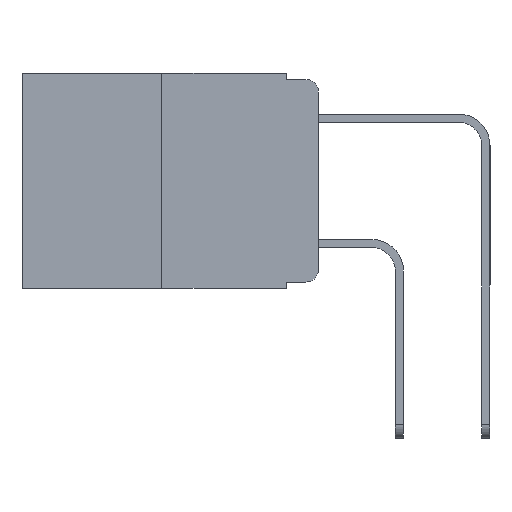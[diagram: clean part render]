
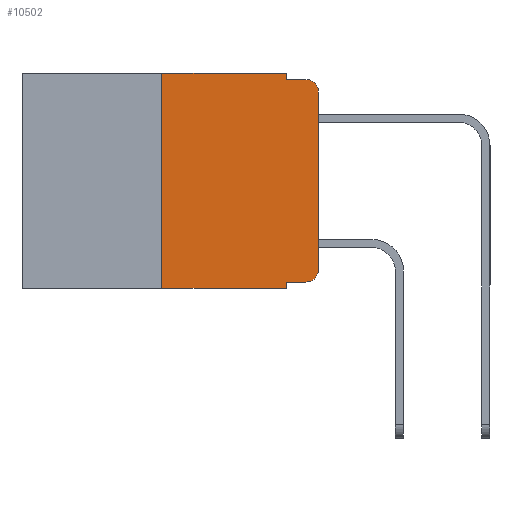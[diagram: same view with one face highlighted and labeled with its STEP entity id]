
A CAD part, left-side view. The second image highlights one B-rep face of the part: STEP entity #10502.
In plain terms, the highlighted planar face has unit normal (-1, 0, 0).
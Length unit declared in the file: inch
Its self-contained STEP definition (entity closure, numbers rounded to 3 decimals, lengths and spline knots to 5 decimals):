
#262 = VERTEX_POINT ( 'NONE', #4031 ) ;
#835 = AXIS2_PLACEMENT_3D ( 'NONE', #12959, #4349, #14311 ) ;
#1050 = EDGE_CURVE ( 'NONE', #7616, #10797, #11537, .T. ) ;
#1137 = ORIENTED_EDGE ( 'NONE', *, *, #1050, .T. ) ;
#1173 = VECTOR ( 'NONE', #4439, 39.37008 ) ;
#1367 = ORIENTED_EDGE ( 'NONE', *, *, #9805, .T. ) ;
#1378 = VECTOR ( 'NONE', #11818, 39.37008 ) ;
#1384 = CARTESIAN_POINT ( 'NONE',  ( 0., 0.051, -0.01 ) ) ;
#1385 = ORIENTED_EDGE ( 'NONE', *, *, #4034, .F. ) ;
#1563 = ORIENTED_EDGE ( 'NONE', *, *, #1939, .F. ) ;
#1656 = VERTEX_POINT ( 'NONE', #17133 ) ;
#1939 = EDGE_CURVE ( 'NONE', #262, #3800, #18120, .T. ) ;
#1963 = ORIENTED_EDGE ( 'NONE', *, *, #16068, .F. ) ;
#2036 = ORIENTED_EDGE ( 'NONE', *, *, #3924, .F. ) ;
#2213 = CARTESIAN_POINT ( 'NONE',  ( 0., 0.02, -0.03 ) ) ;
#2733 = DIRECTION ( 'NONE',  ( 0., 0., -1. ) ) ;
#2740 = CARTESIAN_POINT ( 'NONE',  ( 0., 0., -0.03 ) ) ;
#2903 = VERTEX_POINT ( 'NONE', #16286 ) ;
#3052 = CARTESIAN_POINT ( 'NONE',  ( 0., 0.02, -0.01 ) ) ;
#3535 = VECTOR ( 'NONE', #12997, 39.37008 ) ;
#3647 = ORIENTED_EDGE ( 'NONE', *, *, #4563, .T. ) ;
#3700 = DIRECTION ( 'NONE',  ( 0., 0., -1. ) ) ;
#3800 = VERTEX_POINT ( 'NONE', #13841 ) ;
#3924 = EDGE_CURVE ( 'NONE', #4226, #14583, #13193, .T. ) ;
#3977 = EDGE_LOOP ( 'NONE', ( #1137, #1367, #1385, #1563, #1963, #2036, #3647, #5380, #5435, #6147 ) ) ;
#4031 = CARTESIAN_POINT ( 'NONE',  ( 0., 0.051, 0. ) ) ;
#4034 = EDGE_CURVE ( 'NONE', #3800, #18426, #17832, .T. ) ;
#4226 = VERTEX_POINT ( 'NONE', #15830 ) ;
#4272 = VERTEX_POINT ( 'NONE', #17356 ) ;
#4321 = CARTESIAN_POINT ( 'NONE',  ( 0., 0.473, 0. ) ) ;
#4349 = DIRECTION ( 'NONE',  ( -1., 0., 0. ) ) ;
#4439 = DIRECTION ( 'NONE',  ( 0., 0., 1. ) ) ;
#4563 = EDGE_CURVE ( 'NONE', #4226, #2903, #10103, .T. ) ;
#5380 = ORIENTED_EDGE ( 'NONE', *, *, #12021, .F. ) ;
#5435 = ORIENTED_EDGE ( 'NONE', *, *, #10126, .T. ) ;
#5773 = FACE_OUTER_BOUND ( 'NONE', #3977, .T. ) ;
#5792 = LINE ( 'NONE', #15843, #1378 ) ;
#5847 = CARTESIAN_POINT ( 'NONE',  ( 0., 0.25, 0. ) ) ;
#6147 = ORIENTED_EDGE ( 'NONE', *, *, #8190, .T. ) ;
#6452 = PLANE ( 'NONE',  #9149 ) ;
#7247 = VECTOR ( 'NONE', #13057, 39.37008 ) ;
#7616 = VERTEX_POINT ( 'NONE', #9065 ) ;
#7899 = DIRECTION ( 'NONE',  ( 1., 0., 0. ) ) ;
#8190 = EDGE_CURVE ( 'NONE', #1656, #7616, #10631, .T. ) ;
#9065 = CARTESIAN_POINT ( 'NONE',  ( 0., 0., -0.313 ) ) ;
#9149 = AXIS2_PLACEMENT_3D ( 'NONE', #16229, #7899, #17602 ) ;
#9663 = VECTOR ( 'NONE', #18218, 39.37008 ) ;
#9805 = EDGE_CURVE ( 'NONE', #10797, #18426, #17620, .T. ) ;
#10103 = LINE ( 'NONE', #11979, #9663 ) ;
#10126 = EDGE_CURVE ( 'NONE', #4272, #1656, #5792, .T. ) ;
#10502 = ADVANCED_FACE ( 'NONE', ( #5773 ), #6452, .F. ) ;
#10631 = CIRCLE ( 'NONE', #835, 0.02 ) ;
#10797 = VERTEX_POINT ( 'NONE', #2740 ) ;
#11307 = VECTOR ( 'NONE', #2733, 39.37008 ) ;
#11537 = LINE ( 'NONE', #12613, #7247 ) ;
#11818 = DIRECTION ( 'NONE',  ( 0., -1., 0. ) ) ;
#11979 = CARTESIAN_POINT ( 'NONE',  ( 0., 0.473, -0.343 ) ) ;
#12021 = EDGE_CURVE ( 'NONE', #4272, #2903, #17353, .T. ) ;
#12149 = LINE ( 'NONE', #4321, #3535 ) ;
#12363 = DIRECTION ( 'NONE',  ( -1., 0., 0. ) ) ;
#12613 = CARTESIAN_POINT ( 'NONE',  ( 0., 0., 0. ) ) ;
#12959 = CARTESIAN_POINT ( 'NONE',  ( 0., 0.02, -0.313 ) ) ;
#12997 = DIRECTION ( 'NONE',  ( 0., -1., 0. ) ) ;
#13057 = DIRECTION ( 'NONE',  ( 0., 0., 1. ) ) ;
#13193 = LINE ( 'NONE', #5847, #1173 ) ;
#13337 = VECTOR ( 'NONE', #16649, 39.37008 ) ;
#13586 = AXIS2_PLACEMENT_3D ( 'NONE', #2213, #12363, #3700 ) ;
#13753 = CARTESIAN_POINT ( 'NONE',  ( 0., 0.25, 0. ) ) ;
#13841 = CARTESIAN_POINT ( 'NONE',  ( 0., 0.051, -0.01 ) ) ;
#14233 = VECTOR ( 'NONE', #14489, 39.37008 ) ;
#14311 = DIRECTION ( 'NONE',  ( 0., 0., -1. ) ) ;
#14489 = DIRECTION ( 'NONE',  ( 0., -1., 0. ) ) ;
#14583 = VERTEX_POINT ( 'NONE', #13753 ) ;
#15342 = CARTESIAN_POINT ( 'NONE',  ( 0., 0.051, 0. ) ) ;
#15830 = CARTESIAN_POINT ( 'NONE',  ( 0., 0.25, -0.343 ) ) ;
#15843 = CARTESIAN_POINT ( 'NONE',  ( 0., 0.051, -0.333 ) ) ;
#16068 = EDGE_CURVE ( 'NONE', #14583, #262, #12149, .T. ) ;
#16090 = CARTESIAN_POINT ( 'NONE',  ( 0., 0.051, 0. ) ) ;
#16229 = CARTESIAN_POINT ( 'NONE',  ( 0., 0.473, 0. ) ) ;
#16286 = CARTESIAN_POINT ( 'NONE',  ( 0., 0.051, -0.343 ) ) ;
#16649 = DIRECTION ( 'NONE',  ( 0., 0., -1. ) ) ;
#17133 = CARTESIAN_POINT ( 'NONE',  ( 0., 0.02, -0.333 ) ) ;
#17353 = LINE ( 'NONE', #15342, #13337 ) ;
#17356 = CARTESIAN_POINT ( 'NONE',  ( 0., 0.051, -0.333 ) ) ;
#17602 = DIRECTION ( 'NONE',  ( 0., 0., -1. ) ) ;
#17620 = CIRCLE ( 'NONE', #13586, 0.02 ) ;
#17832 = LINE ( 'NONE', #1384, #14233 ) ;
#18120 = LINE ( 'NONE', #16090, #11307 ) ;
#18218 = DIRECTION ( 'NONE',  ( 0., -1., 0. ) ) ;
#18426 = VERTEX_POINT ( 'NONE', #3052 ) ;
